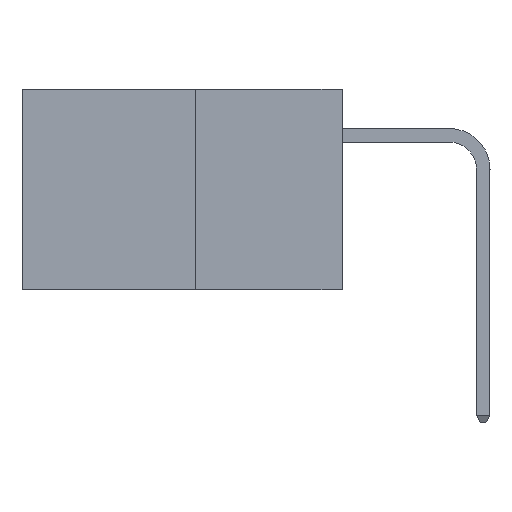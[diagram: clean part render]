
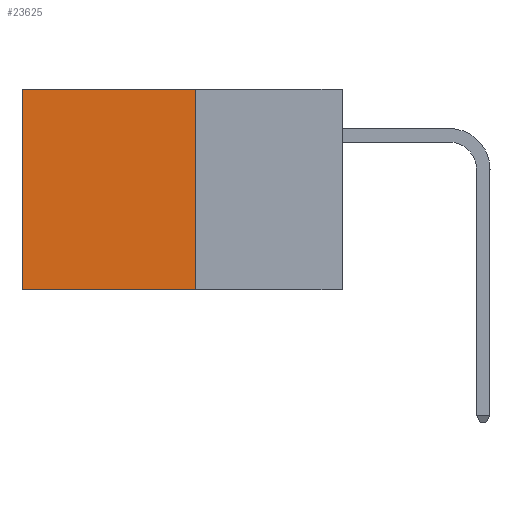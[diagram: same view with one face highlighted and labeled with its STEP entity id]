
A CAD part, left-side view. The second image highlights one B-rep face of the part: STEP entity #23625.
In plain terms, the highlighted planar face has unit normal (-1, 0, 0).
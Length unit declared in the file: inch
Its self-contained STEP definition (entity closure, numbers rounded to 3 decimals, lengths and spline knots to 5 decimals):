
#752 = AXIS2_PLACEMENT_3D ( 'NONE', #8579, #10492, #24069 ) ;
#833 = DIRECTION ( 'NONE',  ( 0., 1., 0. ) ) ;
#1646 = EDGE_CURVE ( 'NONE', #11887, #15024, #9069, .T. ) ;
#2068 = CARTESIAN_POINT ( 'NONE',  ( 0.277, 0.59, 0. ) ) ;
#2590 = ORIENTED_EDGE ( 'NONE', *, *, #23741, .F. ) ;
#3046 = ORIENTED_EDGE ( 'NONE', *, *, #13192, .T. ) ;
#3368 = VERTEX_POINT ( 'NONE', #25379 ) ;
#3788 = VECTOR ( 'NONE', #833, 39.37008 ) ;
#6281 = FACE_OUTER_BOUND ( 'NONE', #11575, .T. ) ;
#8579 = CARTESIAN_POINT ( 'NONE',  ( 0.277, 0.27, -0.37 ) ) ;
#8853 = DIRECTION ( 'NONE',  ( 0., 1., 0. ) ) ;
#9069 = LINE ( 'NONE', #20376, #23910 ) ;
#9933 = DIRECTION ( 'NONE',  ( 0., 0., -1. ) ) ;
#10492 = DIRECTION ( 'NONE',  ( 1., 0., 0. ) ) ;
#11575 = EDGE_LOOP ( 'NONE', ( #14579, #2590, #20502, #3046 ) ) ;
#11844 = CARTESIAN_POINT ( 'NONE',  ( 0.277, 0.27, 0. ) ) ;
#11887 = VERTEX_POINT ( 'NONE', #2068 ) ;
#12199 = CARTESIAN_POINT ( 'NONE',  ( 0.277, 0.59, -0.37 ) ) ;
#13192 = EDGE_CURVE ( 'NONE', #18950, #11887, #19000, .T. ) ;
#13558 = EDGE_CURVE ( 'NONE', #18950, #3368, #24630, .T. ) ;
#14333 = VECTOR ( 'NONE', #9933, 39.37008 ) ;
#14579 = ORIENTED_EDGE ( 'NONE', *, *, #1646, .T. ) ;
#15024 = VERTEX_POINT ( 'NONE', #12199 ) ;
#15709 = CARTESIAN_POINT ( 'NONE',  ( 0.277, 0.27, -0.37 ) ) ;
#16568 = CARTESIAN_POINT ( 'NONE',  ( 0.277, 0.27, -0.37 ) ) ;
#17759 = VECTOR ( 'NONE', #8853, 39.37008 ) ;
#18950 = VERTEX_POINT ( 'NONE', #11844 ) ;
#19000 = LINE ( 'NONE', #20598, #17759 ) ;
#20248 = PLANE ( 'NONE',  #752 ) ;
#20376 = CARTESIAN_POINT ( 'NONE',  ( 0.277, 0.59, -0.37 ) ) ;
#20502 = ORIENTED_EDGE ( 'NONE', *, *, #13558, .F. ) ;
#20519 = DIRECTION ( 'NONE',  ( 0., 0., -1. ) ) ;
#20598 = CARTESIAN_POINT ( 'NONE',  ( 0.277, 0.27, 0. ) ) ;
#23625 = ADVANCED_FACE ( 'NONE', ( #6281 ), #20248, .F. ) ;
#23741 = EDGE_CURVE ( 'NONE', #3368, #15024, #24513, .T. ) ;
#23910 = VECTOR ( 'NONE', #20519, 39.37008 ) ;
#24069 = DIRECTION ( 'NONE',  ( 0., 0., -1. ) ) ;
#24513 = LINE ( 'NONE', #16568, #3788 ) ;
#24630 = LINE ( 'NONE', #15709, #14333 ) ;
#25379 = CARTESIAN_POINT ( 'NONE',  ( 0.277, 0.27, -0.37 ) ) ;
